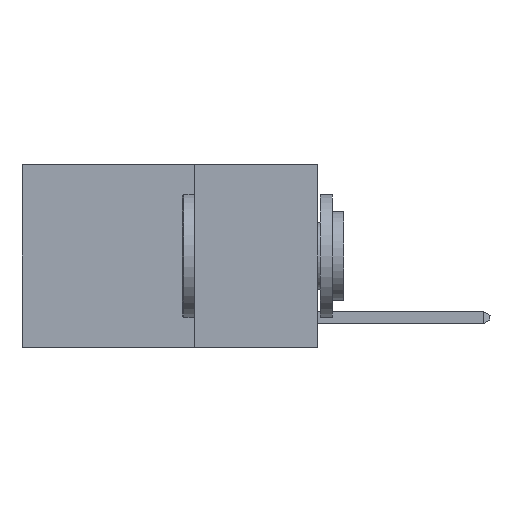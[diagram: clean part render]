
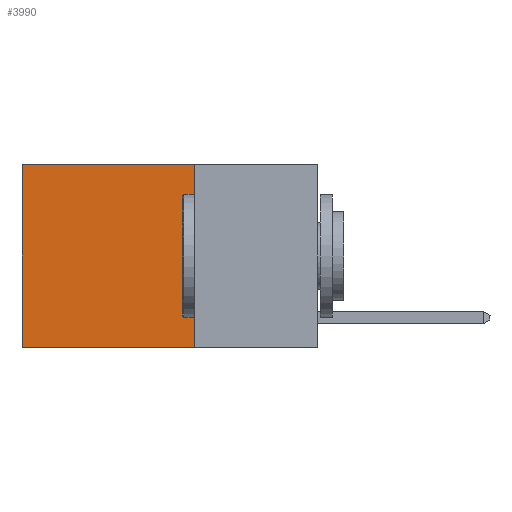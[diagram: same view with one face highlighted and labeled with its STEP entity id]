
A CAD part, left-side view. The second image highlights one B-rep face of the part: STEP entity #3990.
In plain terms, the highlighted planar face has unit normal (-1, 0, 0).
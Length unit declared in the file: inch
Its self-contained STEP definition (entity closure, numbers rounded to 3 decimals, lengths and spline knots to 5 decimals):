
#148 = LINE ( 'NONE', #9189, #2502 ) ;
#666 = CARTESIAN_POINT ( 'NONE',  ( 0.2625, 0.25, 0. ) ) ;
#1148 = DIRECTION ( 'NONE',  ( 1., 0., 0. ) ) ;
#1382 = CARTESIAN_POINT ( 'NONE',  ( 0.2625, 0.25, 0. ) ) ;
#1512 = VECTOR ( 'NONE', #10816, 39.37008 ) ;
#1988 = EDGE_CURVE ( 'NONE', #10721, #10148, #11851, .T. ) ;
#2403 = EDGE_CURVE ( 'NONE', #9269, #10721, #8015, .T. ) ;
#2502 = VECTOR ( 'NONE', #6300, 39.37008 ) ;
#2891 = ORIENTED_EDGE ( 'NONE', *, *, #1988, .T. ) ;
#2963 = VECTOR ( 'NONE', #8200, 39.37008 ) ;
#3223 = CARTESIAN_POINT ( 'NONE',  ( 0.2625, 0.6, -0.37 ) ) ;
#3990 = ADVANCED_FACE ( 'NONE', ( #5952 ), #4896, .F. ) ;
#4384 = AXIS2_PLACEMENT_3D ( 'NONE', #1382, #1148, #4841 ) ;
#4571 = ORIENTED_EDGE ( 'NONE', *, *, #6698, .F. ) ;
#4841 = DIRECTION ( 'NONE',  ( 0., 0., -1. ) ) ;
#4896 = PLANE ( 'NONE',  #4384 ) ;
#5132 = CARTESIAN_POINT ( 'NONE',  ( 0.2625, 0.25, -0.37 ) ) ;
#5409 = EDGE_LOOP ( 'NONE', ( #2891, #4571, #10400, #11818 ) ) ;
#5952 = FACE_OUTER_BOUND ( 'NONE', #5409, .T. ) ;
#6300 = DIRECTION ( 'NONE',  ( 0., 1., 0. ) ) ;
#6698 = EDGE_CURVE ( 'NONE', #9272, #10148, #148, .T. ) ;
#7348 = LINE ( 'NONE', #666, #2963 ) ;
#7401 = CARTESIAN_POINT ( 'NONE',  ( 0.2625, 0.6, 0. ) ) ;
#8015 = LINE ( 'NONE', #8075, #1512 ) ;
#8075 = CARTESIAN_POINT ( 'NONE',  ( 0.2625, 0.25, 0. ) ) ;
#8200 = DIRECTION ( 'NONE',  ( 0., 0., -1. ) ) ;
#9189 = CARTESIAN_POINT ( 'NONE',  ( 0.2625, 0.25, -0.37 ) ) ;
#9269 = VERTEX_POINT ( 'NONE', #9986 ) ;
#9272 = VERTEX_POINT ( 'NONE', #5132 ) ;
#9774 = DIRECTION ( 'NONE',  ( 0., 0., -1. ) ) ;
#9986 = CARTESIAN_POINT ( 'NONE',  ( 0.2625, 0.25, 0. ) ) ;
#10148 = VERTEX_POINT ( 'NONE', #3223 ) ;
#10400 = ORIENTED_EDGE ( 'NONE', *, *, #12069, .F. ) ;
#10721 = VERTEX_POINT ( 'NONE', #7401 ) ;
#10816 = DIRECTION ( 'NONE',  ( 0., 1., 0. ) ) ;
#11094 = VECTOR ( 'NONE', #9774, 39.37008 ) ;
#11678 = CARTESIAN_POINT ( 'NONE',  ( 0.2625, 0.6, 0. ) ) ;
#11818 = ORIENTED_EDGE ( 'NONE', *, *, #2403, .T. ) ;
#11851 = LINE ( 'NONE', #11678, #11094 ) ;
#12069 = EDGE_CURVE ( 'NONE', #9269, #9272, #7348, .T. ) ;
